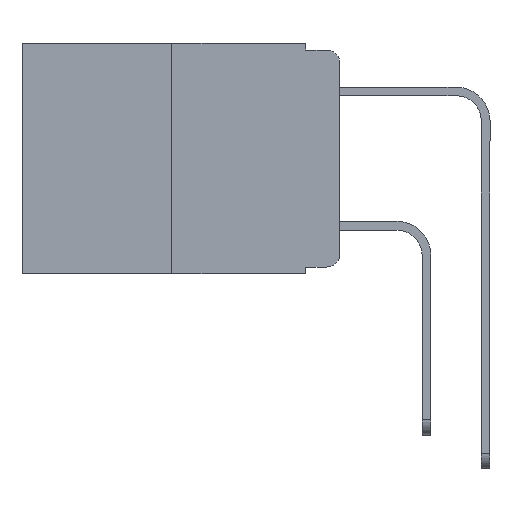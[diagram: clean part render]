
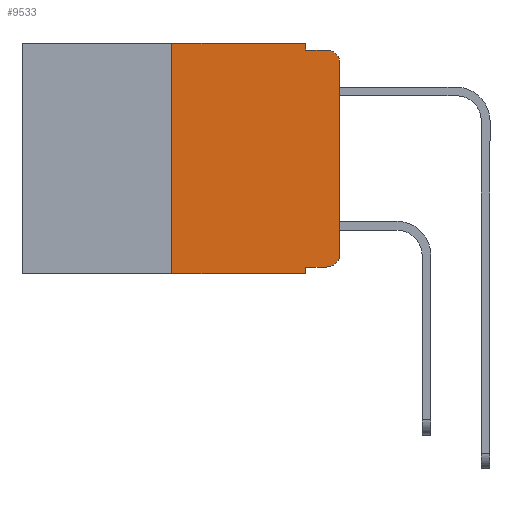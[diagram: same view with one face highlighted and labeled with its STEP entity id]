
A CAD part, left-side view. The second image highlights one B-rep face of the part: STEP entity #9533.
In plain terms, the highlighted planar face has unit normal (-1, 0, 0).
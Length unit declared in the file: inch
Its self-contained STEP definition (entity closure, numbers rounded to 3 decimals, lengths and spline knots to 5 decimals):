
#102 = CARTESIAN_POINT ( 'NONE',  ( 0., 0.25, -0.343 ) ) ;
#269 = EDGE_CURVE ( 'NONE', #5207, #9036, #9958, .T. ) ;
#733 = CARTESIAN_POINT ( 'NONE',  ( 0., 0.051, -0.01 ) ) ;
#774 = CARTESIAN_POINT ( 'NONE',  ( 0., 0.051, -0.333 ) ) ;
#866 = CARTESIAN_POINT ( 'NONE',  ( 0., 0.051, 0. ) ) ;
#937 = VECTOR ( 'NONE', #3915, 39.37008 ) ;
#945 = CARTESIAN_POINT ( 'NONE',  ( 0., 0., -0.03 ) ) ;
#1051 = DIRECTION ( 'NONE',  ( 0., 0., -1. ) ) ;
#1057 = DIRECTION ( 'NONE',  ( 0., 0., 1. ) ) ;
#1135 = VECTOR ( 'NONE', #4189, 39.37008 ) ;
#1344 = VERTEX_POINT ( 'NONE', #945 ) ;
#1478 = LINE ( 'NONE', #11458, #1135 ) ;
#1525 = VERTEX_POINT ( 'NONE', #774 ) ;
#1815 = LINE ( 'NONE', #2153, #11271 ) ;
#2153 = CARTESIAN_POINT ( 'NONE',  ( 0., 0.25, 0. ) ) ;
#2267 = VERTEX_POINT ( 'NONE', #733 ) ;
#2661 = AXIS2_PLACEMENT_3D ( 'NONE', #12387, #6964, #1051 ) ;
#2874 = VERTEX_POINT ( 'NONE', #866 ) ;
#2965 = EDGE_LOOP ( 'NONE', ( #5264, #10784, #12194, #8828, #8174, #7629, #4422, #4147, #3984, #3543 ) ) ;
#3465 = LINE ( 'NONE', #10419, #8752 ) ;
#3543 = ORIENTED_EDGE ( 'NONE', *, *, #4958, .T. ) ;
#3915 = DIRECTION ( 'NONE',  ( 0., -1., 0. ) ) ;
#3984 = ORIENTED_EDGE ( 'NONE', *, *, #5580, .T. ) ;
#4147 = ORIENTED_EDGE ( 'NONE', *, *, #6212, .F. ) ;
#4189 = DIRECTION ( 'NONE',  ( 0., 0., -1. ) ) ;
#4422 = ORIENTED_EDGE ( 'NONE', *, *, #269, .T. ) ;
#4646 = VERTEX_POINT ( 'NONE', #6611 ) ;
#4688 = VERTEX_POINT ( 'NONE', #5748 ) ;
#4773 = CIRCLE ( 'NONE', #2661, 0.02 ) ;
#4928 = CARTESIAN_POINT ( 'NONE',  ( 0., 0.051, -0.333 ) ) ;
#4958 = EDGE_CURVE ( 'NONE', #4688, #12324, #6034, .T. ) ;
#5115 = CARTESIAN_POINT ( 'NONE',  ( 0., 0.25, 0. ) ) ;
#5207 = VERTEX_POINT ( 'NONE', #102 ) ;
#5264 = ORIENTED_EDGE ( 'NONE', *, *, #9278, .T. ) ;
#5403 = AXIS2_PLACEMENT_3D ( 'NONE', #5795, #12159, #6739 ) ;
#5481 = LINE ( 'NONE', #7917, #11639 ) ;
#5516 = DIRECTION ( 'NONE',  ( 1., 0., 0. ) ) ;
#5580 = EDGE_CURVE ( 'NONE', #1525, #4688, #10738, .T. ) ;
#5748 = CARTESIAN_POINT ( 'NONE',  ( 0., 0.02, -0.333 ) ) ;
#5795 = CARTESIAN_POINT ( 'NONE',  ( 0., 0.02, -0.313 ) ) ;
#5814 = CARTESIAN_POINT ( 'NONE',  ( 0., 0.473, -0.343 ) ) ;
#5864 = VECTOR ( 'NONE', #8621, 39.37008 ) ;
#6034 = CIRCLE ( 'NONE', #5403, 0.02 ) ;
#6212 = EDGE_CURVE ( 'NONE', #1525, #9036, #3465, .T. ) ;
#6472 = AXIS2_PLACEMENT_3D ( 'NONE', #7311, #5516, #11898 ) ;
#6611 = CARTESIAN_POINT ( 'NONE',  ( 0., 0.02, -0.01 ) ) ;
#6739 = DIRECTION ( 'NONE',  ( 0., 0., -1. ) ) ;
#6839 = EDGE_CURVE ( 'NONE', #5207, #7468, #1815, .T. ) ;
#6964 = DIRECTION ( 'NONE',  ( -1., 0., 0. ) ) ;
#7311 = CARTESIAN_POINT ( 'NONE',  ( 0., 0.473, 0. ) ) ;
#7459 = EDGE_CURVE ( 'NONE', #2874, #2267, #1478, .T. ) ;
#7468 = VERTEX_POINT ( 'NONE', #5115 ) ;
#7504 = DIRECTION ( 'NONE',  ( 0., -1., 0. ) ) ;
#7546 = VECTOR ( 'NONE', #7504, 39.37008 ) ;
#7564 = LINE ( 'NONE', #11124, #12073 ) ;
#7629 = ORIENTED_EDGE ( 'NONE', *, *, #6839, .F. ) ;
#7770 = CARTESIAN_POINT ( 'NONE',  ( 0., 0., -0.313 ) ) ;
#7917 = CARTESIAN_POINT ( 'NONE',  ( 0., 0., 0. ) ) ;
#8057 = EDGE_CURVE ( 'NONE', #2267, #4646, #11395, .T. ) ;
#8174 = ORIENTED_EDGE ( 'NONE', *, *, #11196, .F. ) ;
#8460 = CARTESIAN_POINT ( 'NONE',  ( 0., 0.051, -0.343 ) ) ;
#8621 = DIRECTION ( 'NONE',  ( 0., -1., 0. ) ) ;
#8694 = EDGE_CURVE ( 'NONE', #1344, #4646, #4773, .T. ) ;
#8752 = VECTOR ( 'NONE', #11325, 39.37008 ) ;
#8828 = ORIENTED_EDGE ( 'NONE', *, *, #7459, .F. ) ;
#8849 = DIRECTION ( 'NONE',  ( 0., 0., 1. ) ) ;
#9036 = VERTEX_POINT ( 'NONE', #8460 ) ;
#9187 = PLANE ( 'NONE',  #6472 ) ;
#9278 = EDGE_CURVE ( 'NONE', #12324, #1344, #5481, .T. ) ;
#9533 = ADVANCED_FACE ( 'NONE', ( #11491 ), #9187, .F. ) ;
#9958 = LINE ( 'NONE', #5814, #7546 ) ;
#10196 = DIRECTION ( 'NONE',  ( 0., -1., 0. ) ) ;
#10372 = CARTESIAN_POINT ( 'NONE',  ( 0., 0.051, -0.01 ) ) ;
#10419 = CARTESIAN_POINT ( 'NONE',  ( 0., 0.051, 0. ) ) ;
#10738 = LINE ( 'NONE', #4928, #5864 ) ;
#10784 = ORIENTED_EDGE ( 'NONE', *, *, #8694, .T. ) ;
#11124 = CARTESIAN_POINT ( 'NONE',  ( 0., 0.473, 0. ) ) ;
#11196 = EDGE_CURVE ( 'NONE', #7468, #2874, #7564, .T. ) ;
#11271 = VECTOR ( 'NONE', #1057, 39.37008 ) ;
#11325 = DIRECTION ( 'NONE',  ( 0., 0., -1. ) ) ;
#11395 = LINE ( 'NONE', #10372, #937 ) ;
#11458 = CARTESIAN_POINT ( 'NONE',  ( 0., 0.051, 0. ) ) ;
#11491 = FACE_OUTER_BOUND ( 'NONE', #2965, .T. ) ;
#11639 = VECTOR ( 'NONE', #8849, 39.37008 ) ;
#11898 = DIRECTION ( 'NONE',  ( 0., 0., -1. ) ) ;
#12073 = VECTOR ( 'NONE', #10196, 39.37008 ) ;
#12159 = DIRECTION ( 'NONE',  ( -1., 0., 0. ) ) ;
#12194 = ORIENTED_EDGE ( 'NONE', *, *, #8057, .F. ) ;
#12324 = VERTEX_POINT ( 'NONE', #7770 ) ;
#12387 = CARTESIAN_POINT ( 'NONE',  ( 0., 0.02, -0.03 ) ) ;
